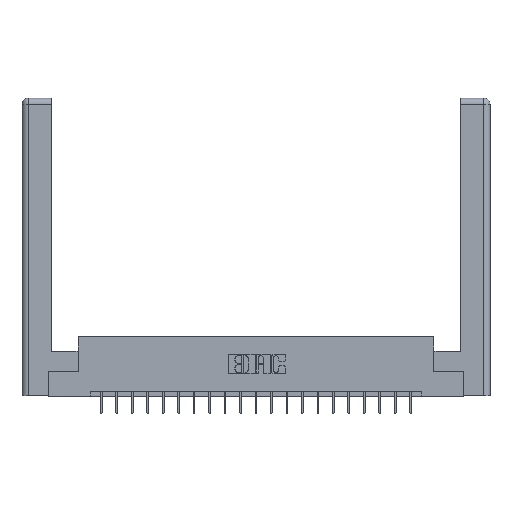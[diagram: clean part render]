
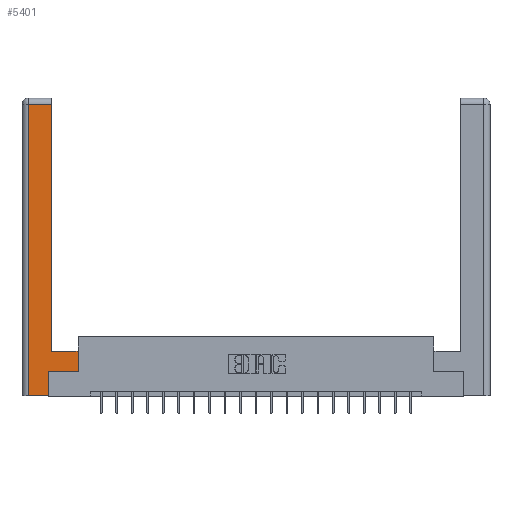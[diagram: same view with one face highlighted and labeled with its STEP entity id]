
A CAD part, top view. The second image highlights one B-rep face of the part: STEP entity #5401.
In plain terms, the highlighted planar face has unit normal (0, 0, 1).
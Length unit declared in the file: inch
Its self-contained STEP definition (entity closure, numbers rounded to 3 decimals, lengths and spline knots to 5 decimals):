
#580 = CARTESIAN_POINT ( 'NONE',  ( 0.0615, 2.94, 0. ) ) ;
#1187 = EDGE_CURVE ( 'NONE', #8893, #16925, #5437, .T. ) ;
#1759 = VECTOR ( 'NONE', #13367, 39.37008 ) ;
#2030 = VECTOR ( 'NONE', #9444, 39.37008 ) ;
#2755 = LINE ( 'NONE', #19691, #14372 ) ;
#3062 = CARTESIAN_POINT ( 'NONE',  ( 0.565, 0.45, 0. ) ) ;
#3188 = EDGE_CURVE ( 'NONE', #12698, #19612, #20184, .T. ) ;
#3318 = VECTOR ( 'NONE', #20991, 39.37008 ) ;
#3358 = VECTOR ( 'NONE', #11012, 39.37008 ) ;
#3728 = CARTESIAN_POINT ( 'NONE',  ( 0.295, 3., 0. ) ) ;
#3862 = ORIENTED_EDGE ( 'NONE', *, *, #1187, .T. ) ;
#3994 = EDGE_CURVE ( 'NONE', #10966, #11898, #17507, .T. ) ;
#4144 = EDGE_CURVE ( 'NONE', #5057, #8893, #7779, .T. ) ;
#4523 = EDGE_CURVE ( 'NONE', #14727, #10966, #21424, .T. ) ;
#4807 = CARTESIAN_POINT ( 'NONE',  ( 0.265, 0., 0. ) ) ;
#5057 = VERTEX_POINT ( 'NONE', #580 ) ;
#5401 = ADVANCED_FACE ( 'NONE', ( #7847 ), #9409, .F. ) ;
#5437 = LINE ( 'NONE', #4807, #1759 ) ;
#5738 = EDGE_CURVE ( 'NONE', #19612, #14727, #2755, .T. ) ;
#6257 = ORIENTED_EDGE ( 'NONE', *, *, #5738, .T. ) ;
#7563 = CARTESIAN_POINT ( 'NONE',  ( 0.295, 0.45, 0. ) ) ;
#7779 = LINE ( 'NONE', #14293, #9644 ) ;
#7847 = FACE_OUTER_BOUND ( 'NONE', #8374, .T. ) ;
#7899 = CARTESIAN_POINT ( 'NONE',  ( 0.565, 0.245, 0. ) ) ;
#7977 = ORIENTED_EDGE ( 'NONE', *, *, #13116, .T. ) ;
#8374 = EDGE_LOOP ( 'NONE', ( #9172, #21283, #14636, #3862, #7977, #15367, #6257, #13577 ) ) ;
#8893 = VERTEX_POINT ( 'NONE', #12479 ) ;
#9134 = DIRECTION ( 'NONE',  ( 0., -1., 0. ) ) ;
#9172 = ORIENTED_EDGE ( 'NONE', *, *, #3994, .T. ) ;
#9409 = PLANE ( 'NONE',  #11639 ) ;
#9444 = DIRECTION ( 'NONE',  ( 0., 1., 0. ) ) ;
#9644 = VECTOR ( 'NONE', #9134, 39.37008 ) ;
#10611 = DIRECTION ( 'NONE',  ( -1., 0., 0. ) ) ;
#10966 = VERTEX_POINT ( 'NONE', #16588 ) ;
#11012 = DIRECTION ( 'NONE',  ( 1., 0., 0. ) ) ;
#11048 = DIRECTION ( 'NONE',  ( 0., 0., -1. ) ) ;
#11449 = CARTESIAN_POINT ( 'NONE',  ( 0.265, 0.245, 0. ) ) ;
#11639 = AXIS2_PLACEMENT_3D ( 'NONE', #17669, #11048, #20986 ) ;
#11898 = VERTEX_POINT ( 'NONE', #18681 ) ;
#12479 = CARTESIAN_POINT ( 'NONE',  ( 0.0615, 0., 0. ) ) ;
#12698 = VERTEX_POINT ( 'NONE', #11449 ) ;
#13116 = EDGE_CURVE ( 'NONE', #16925, #12698, #18030, .T. ) ;
#13367 = DIRECTION ( 'NONE',  ( 1., 0., 0. ) ) ;
#13577 = ORIENTED_EDGE ( 'NONE', *, *, #4523, .T. ) ;
#13847 = CARTESIAN_POINT ( 'NONE',  ( 0.0615, 2.94, 0. ) ) ;
#14293 = CARTESIAN_POINT ( 'NONE',  ( 0.0615, 0., 0. ) ) ;
#14372 = VECTOR ( 'NONE', #14798, 39.37008 ) ;
#14374 = CARTESIAN_POINT ( 'NONE',  ( 0.265, 0.245, 0. ) ) ;
#14636 = ORIENTED_EDGE ( 'NONE', *, *, #4144, .T. ) ;
#14727 = VERTEX_POINT ( 'NONE', #3062 ) ;
#14798 = DIRECTION ( 'NONE',  ( 0., 1., 0. ) ) ;
#15367 = ORIENTED_EDGE ( 'NONE', *, *, #3188, .T. ) ;
#15784 = VECTOR ( 'NONE', #10611, 39.37008 ) ;
#16588 = CARTESIAN_POINT ( 'NONE',  ( 0.295, 0.45, 0. ) ) ;
#16925 = VERTEX_POINT ( 'NONE', #21302 ) ;
#17361 = LINE ( 'NONE', #13847, #15784 ) ;
#17507 = LINE ( 'NONE', #3728, #18544 ) ;
#17669 = CARTESIAN_POINT ( 'NONE',  ( 0., 0., 0. ) ) ;
#18030 = LINE ( 'NONE', #14374, #2030 ) ;
#18544 = VECTOR ( 'NONE', #20629, 39.37008 ) ;
#18681 = CARTESIAN_POINT ( 'NONE',  ( 0.295, 2.94, 0. ) ) ;
#18816 = EDGE_CURVE ( 'NONE', #11898, #5057, #17361, .T. ) ;
#19131 = CARTESIAN_POINT ( 'NONE',  ( 0.565, 0.245, 0. ) ) ;
#19612 = VERTEX_POINT ( 'NONE', #19131 ) ;
#19691 = CARTESIAN_POINT ( 'NONE',  ( 0.565, 0.45, 0. ) ) ;
#20184 = LINE ( 'NONE', #7899, #3358 ) ;
#20629 = DIRECTION ( 'NONE',  ( 0., 1., 0. ) ) ;
#20986 = DIRECTION ( 'NONE',  ( -1., 0., 0. ) ) ;
#20991 = DIRECTION ( 'NONE',  ( -1., 0., 0. ) ) ;
#21283 = ORIENTED_EDGE ( 'NONE', *, *, #18816, .T. ) ;
#21302 = CARTESIAN_POINT ( 'NONE',  ( 0.265, 0., 0. ) ) ;
#21424 = LINE ( 'NONE', #7563, #3318 ) ;
